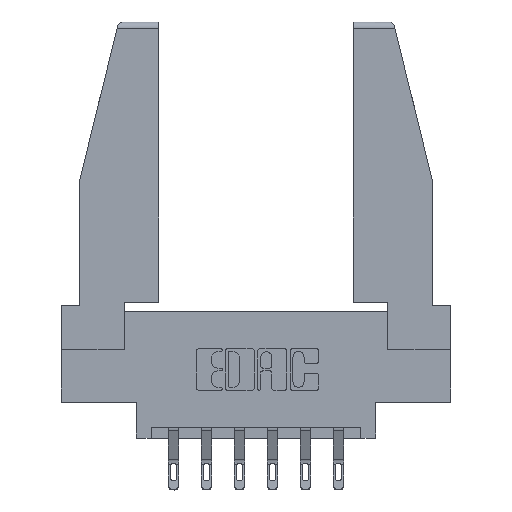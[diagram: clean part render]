
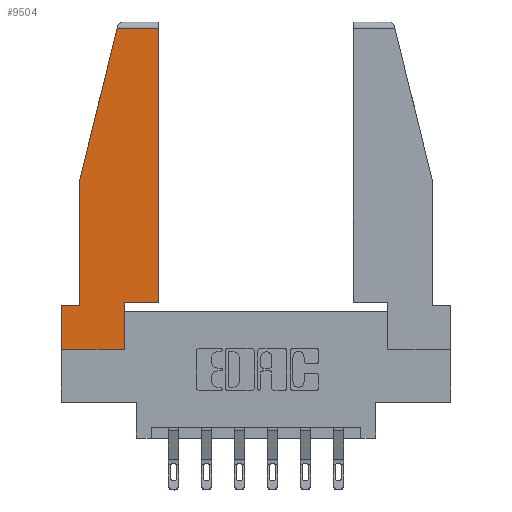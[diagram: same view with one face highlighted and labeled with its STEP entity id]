
A CAD part, top view. The second image highlights one B-rep face of the part: STEP entity #9504.
In plain terms, the highlighted planar face has unit normal (0, 0, 1).
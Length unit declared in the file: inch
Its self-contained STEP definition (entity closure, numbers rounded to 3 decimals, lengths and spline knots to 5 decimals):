
#350 = VERTEX_POINT ( 'NONE', #8533 ) ;
#641 = EDGE_CURVE ( 'NONE', #1113, #5002, #8797, .T. ) ;
#686 = CARTESIAN_POINT ( 'NONE',  ( 0.086, 0.8, 0. ) ) ;
#803 = ORIENTED_EDGE ( 'NONE', *, *, #891, .T. ) ;
#891 = EDGE_CURVE ( 'NONE', #10811, #350, #8951, .T. ) ;
#1108 = LINE ( 'NONE', #10202, #10848 ) ;
#1113 = VERTEX_POINT ( 'NONE', #7920 ) ;
#1386 = DIRECTION ( 'NONE',  ( 0., 0., 1. ) ) ;
#1664 = DIRECTION ( 'NONE',  ( -0.239, -0.971, 0. ) ) ;
#1881 = VECTOR ( 'NONE', #5663, 39.37008 ) ;
#2140 = VERTEX_POINT ( 'NONE', #10452 ) ;
#2166 = DIRECTION ( 'NONE',  ( 1., 0., 0. ) ) ;
#2526 = ORIENTED_EDGE ( 'NONE', *, *, #5424, .T. ) ;
#3098 = VECTOR ( 'NONE', #2166, 39.37008 ) ;
#3131 = ORIENTED_EDGE ( 'NONE', *, *, #641, .T. ) ;
#3304 = DIRECTION ( 'NONE',  ( 1., 0., 0. ) ) ;
#3394 = LINE ( 'NONE', #9021, #3098 ) ;
#3417 = CARTESIAN_POINT ( 'NONE',  ( 0., 0.21, 0. ) ) ;
#3629 = EDGE_CURVE ( 'NONE', #3700, #10811, #9393, .T. ) ;
#3700 = VERTEX_POINT ( 'NONE', #686 ) ;
#3755 = CARTESIAN_POINT ( 'NONE',  ( 0., 0., 0. ) ) ;
#3978 = CARTESIAN_POINT ( 'NONE',  ( 0.297, 0., 0. ) ) ;
#4014 = ORIENTED_EDGE ( 'NONE', *, *, #12090, .T. ) ;
#4386 = DIRECTION ( 'NONE',  ( 0., 1., 0. ) ) ;
#4637 = DIRECTION ( 'NONE',  ( 0., 1., 0. ) ) ;
#5002 = VERTEX_POINT ( 'NONE', #7967 ) ;
#5375 = EDGE_CURVE ( 'NONE', #11636, #10047, #11135, .T. ) ;
#5424 = EDGE_CURVE ( 'NONE', #2140, #1113, #1108, .T. ) ;
#5449 = VECTOR ( 'NONE', #1664, 39.37008 ) ;
#5570 = CARTESIAN_POINT ( 'NONE',  ( 0.297, 0.223, 0. ) ) ;
#5663 = DIRECTION ( 'NONE',  ( -1., 0., 0. ) ) ;
#5968 = CARTESIAN_POINT ( 'NONE',  ( 0., 0., 0. ) ) ;
#6570 = AXIS2_PLACEMENT_3D ( 'NONE', #5968, #1386, #3304 ) ;
#6639 = FACE_OUTER_BOUND ( 'NONE', #7242, .T. ) ;
#6736 = LINE ( 'NONE', #9264, #8081 ) ;
#6921 = LINE ( 'NONE', #3417, #10643 ) ;
#7118 = CARTESIAN_POINT ( 'NONE',  ( 0.086, 0.8, 0. ) ) ;
#7165 = DIRECTION ( 'NONE',  ( -1., 0., 0. ) ) ;
#7168 = VECTOR ( 'NONE', #9002, 39.37008 ) ;
#7242 = EDGE_LOOP ( 'NONE', ( #2526, #3131, #7443, #11674, #803, #7570, #12097, #4014, #11582 ) ) ;
#7429 = EDGE_CURVE ( 'NONE', #350, #11636, #6921, .T. ) ;
#7443 = ORIENTED_EDGE ( 'NONE', *, *, #7516, .T. ) ;
#7516 = EDGE_CURVE ( 'NONE', #5002, #3700, #8259, .T. ) ;
#7570 = ORIENTED_EDGE ( 'NONE', *, *, #7429, .T. ) ;
#7873 = CARTESIAN_POINT ( 'NONE',  ( 0., 0., 0. ) ) ;
#7920 = CARTESIAN_POINT ( 'NONE',  ( 0.461, 1.52, 0. ) ) ;
#7967 = CARTESIAN_POINT ( 'NONE',  ( 0.2636, 1.52, 0. ) ) ;
#8081 = VECTOR ( 'NONE', #4637, 39.37008 ) ;
#8259 = LINE ( 'NONE', #12008, #5449 ) ;
#8525 = CARTESIAN_POINT ( 'NONE',  ( 0., 1.52, 0. ) ) ;
#8533 = CARTESIAN_POINT ( 'NONE',  ( 0., 0.21, 0. ) ) ;
#8613 = VECTOR ( 'NONE', #9705, 39.37008 ) ;
#8797 = LINE ( 'NONE', #8525, #1881 ) ;
#8951 = LINE ( 'NONE', #9057, #11470 ) ;
#9002 = DIRECTION ( 'NONE',  ( 0., -1., 0. ) ) ;
#9021 = CARTESIAN_POINT ( 'NONE',  ( 0.297, 0.223, 0. ) ) ;
#9057 = CARTESIAN_POINT ( 'NONE',  ( 0., 0.21, 0. ) ) ;
#9078 = VERTEX_POINT ( 'NONE', #5570 ) ;
#9264 = CARTESIAN_POINT ( 'NONE',  ( 0.297, 0., 0. ) ) ;
#9393 = LINE ( 'NONE', #7118, #7168 ) ;
#9504 = ADVANCED_FACE ( 'NONE', ( #6639 ), #11629, .T. ) ;
#9705 = DIRECTION ( 'NONE',  ( 1., 0., 0. ) ) ;
#10047 = VERTEX_POINT ( 'NONE', #3978 ) ;
#10153 = CARTESIAN_POINT ( 'NONE',  ( 0.086, 0.21, 0. ) ) ;
#10202 = CARTESIAN_POINT ( 'NONE',  ( 0.461, 0.223, 0. ) ) ;
#10231 = EDGE_CURVE ( 'NONE', #9078, #2140, #3394, .T. ) ;
#10452 = CARTESIAN_POINT ( 'NONE',  ( 0.461, 0.223, 0. ) ) ;
#10643 = VECTOR ( 'NONE', #11914, 39.37008 ) ;
#10811 = VERTEX_POINT ( 'NONE', #10153 ) ;
#10848 = VECTOR ( 'NONE', #4386, 39.37008 ) ;
#11135 = LINE ( 'NONE', #7873, #8613 ) ;
#11470 = VECTOR ( 'NONE', #7165, 39.37008 ) ;
#11582 = ORIENTED_EDGE ( 'NONE', *, *, #10231, .T. ) ;
#11629 = PLANE ( 'NONE',  #6570 ) ;
#11636 = VERTEX_POINT ( 'NONE', #3755 ) ;
#11674 = ORIENTED_EDGE ( 'NONE', *, *, #3629, .T. ) ;
#11914 = DIRECTION ( 'NONE',  ( 0., -1., 0. ) ) ;
#12008 = CARTESIAN_POINT ( 'NONE',  ( 0.271, 1.55, 0. ) ) ;
#12090 = EDGE_CURVE ( 'NONE', #10047, #9078, #6736, .T. ) ;
#12097 = ORIENTED_EDGE ( 'NONE', *, *, #5375, .T. ) ;
